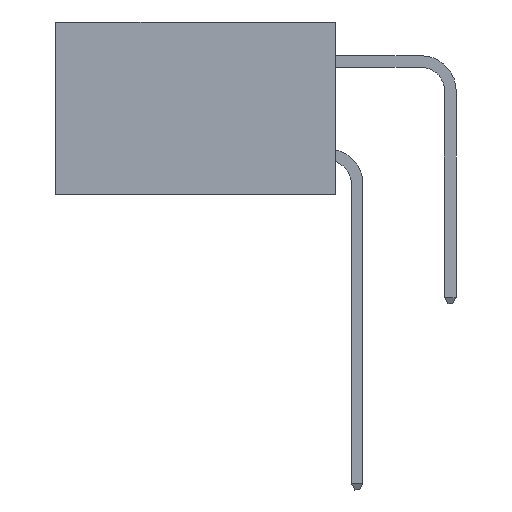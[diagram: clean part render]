
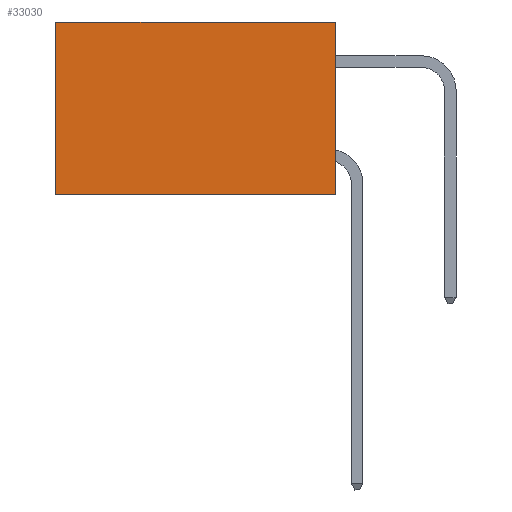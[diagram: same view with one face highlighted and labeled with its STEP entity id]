
A CAD part, left-side view. The second image highlights one B-rep face of the part: STEP entity #33030.
In plain terms, the highlighted planar face has unit normal (-1, 0, 0).
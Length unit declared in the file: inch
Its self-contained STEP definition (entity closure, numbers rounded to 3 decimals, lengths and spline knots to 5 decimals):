
#787 = DIRECTION ( 'NONE',  ( 0., 1., 0. ) ) ;
#1323 = ORIENTED_EDGE ( 'NONE', *, *, #22894, .T. ) ;
#2180 = CARTESIAN_POINT ( 'NONE',  ( 0.2875, 0.6, 0. ) ) ;
#2239 = ORIENTED_EDGE ( 'NONE', *, *, #26771, .T. ) ;
#2357 = LINE ( 'NONE', #11281, #31851 ) ;
#4102 = EDGE_CURVE ( 'NONE', #28173, #18029, #30293, .T. ) ;
#4428 = VECTOR ( 'NONE', #787, 39.37008 ) ;
#6182 = EDGE_CURVE ( 'NONE', #18029, #17594, #2357, .T. ) ;
#7158 = PLANE ( 'NONE',  #20569 ) ;
#10025 = ORIENTED_EDGE ( 'NONE', *, *, #6182, .F. ) ;
#11281 = CARTESIAN_POINT ( 'NONE',  ( 0.2875, 0., -0.37 ) ) ;
#11676 = CARTESIAN_POINT ( 'NONE',  ( 0.2875, 0., -0.37 ) ) ;
#13952 = EDGE_LOOP ( 'NONE', ( #2239, #10025, #23891, #1323 ) ) ;
#17594 = VERTEX_POINT ( 'NONE', #33860 ) ;
#18029 = VERTEX_POINT ( 'NONE', #11676 ) ;
#20569 = AXIS2_PLACEMENT_3D ( 'NONE', #27710, #30692, #36675 ) ;
#21646 = LINE ( 'NONE', #29462, #34137 ) ;
#22894 = EDGE_CURVE ( 'NONE', #28173, #30725, #35359, .T. ) ;
#23891 = ORIENTED_EDGE ( 'NONE', *, *, #4102, .F. ) ;
#24191 = CARTESIAN_POINT ( 'NONE',  ( 0.2875, 0., 0. ) ) ;
#26439 = DIRECTION ( 'NONE',  ( 0., 1., 0. ) ) ;
#26771 = EDGE_CURVE ( 'NONE', #30725, #17594, #21646, .T. ) ;
#27710 = CARTESIAN_POINT ( 'NONE',  ( 0.2875, 0., 0. ) ) ;
#28173 = VERTEX_POINT ( 'NONE', #24191 ) ;
#28425 = VECTOR ( 'NONE', #37804, 39.37008 ) ;
#28706 = CARTESIAN_POINT ( 'NONE',  ( 0.2875, 0., 0. ) ) ;
#29325 = DIRECTION ( 'NONE',  ( 0., 0., -1. ) ) ;
#29462 = CARTESIAN_POINT ( 'NONE',  ( 0.2875, 0.6, 0. ) ) ;
#30293 = LINE ( 'NONE', #28706, #28425 ) ;
#30299 = FACE_OUTER_BOUND ( 'NONE', #13952, .T. ) ;
#30692 = DIRECTION ( 'NONE',  ( 1., 0., 0. ) ) ;
#30725 = VERTEX_POINT ( 'NONE', #2180 ) ;
#31851 = VECTOR ( 'NONE', #26439, 39.37008 ) ;
#33030 = ADVANCED_FACE ( 'NONE', ( #30299 ), #7158, .F. ) ;
#33860 = CARTESIAN_POINT ( 'NONE',  ( 0.2875, 0.6, -0.37 ) ) ;
#34137 = VECTOR ( 'NONE', #29325, 39.37008 ) ;
#35359 = LINE ( 'NONE', #36032, #4428 ) ;
#36032 = CARTESIAN_POINT ( 'NONE',  ( 0.2875, 0., 0. ) ) ;
#36675 = DIRECTION ( 'NONE',  ( 0., 0., -1. ) ) ;
#37804 = DIRECTION ( 'NONE',  ( 0., 0., -1. ) ) ;
